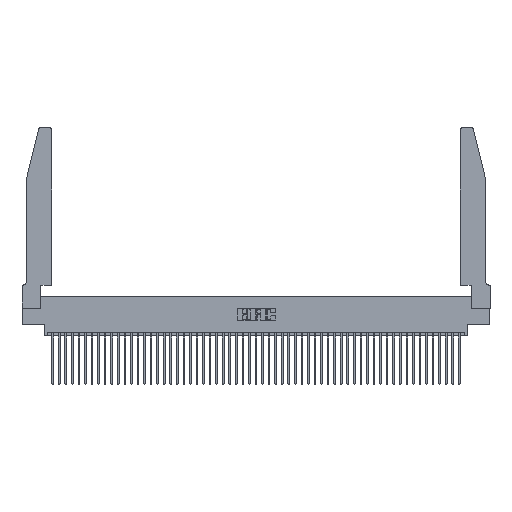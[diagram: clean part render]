
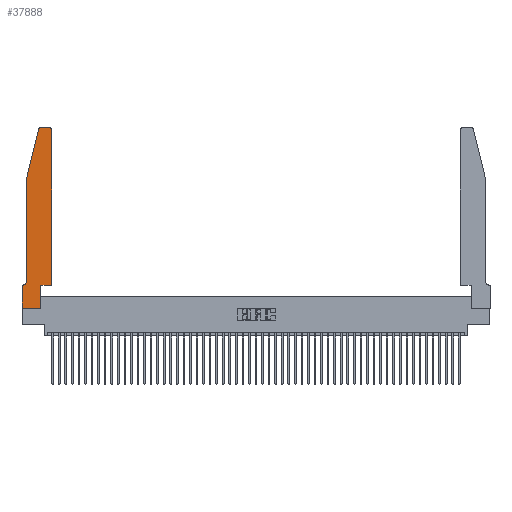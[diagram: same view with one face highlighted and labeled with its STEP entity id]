
A CAD part, top view. The second image highlights one B-rep face of the part: STEP entity #37888.
In plain terms, the highlighted planar face has unit normal (0, 0, 1).
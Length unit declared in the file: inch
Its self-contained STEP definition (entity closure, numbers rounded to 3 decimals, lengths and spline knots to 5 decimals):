
#162 = CARTESIAN_POINT ( 'NONE',  ( 0., 0.35, 0.37 ) ) ;
#283 = VERTEX_POINT ( 'NONE', #8552 ) ;
#716 = VECTOR ( 'NONE', #48132, 39.37008 ) ;
#825 = CARTESIAN_POINT ( 'NONE',  ( 0.25487, 2.72718, 0.37 ) ) ;
#1293 = DIRECTION ( 'NONE',  ( 0., -1., 0. ) ) ;
#2922 = VECTOR ( 'NONE', #34797, 39.37008 ) ;
#3136 = EDGE_CURVE ( 'NONE', #283, #15761, #44044, .T. ) ;
#3512 = VERTEX_POINT ( 'NONE', #41169 ) ;
#4586 = CARTESIAN_POINT ( 'NONE',  ( 0.4505, 0.35, 0.37 ) ) ;
#4816 = AXIS2_PLACEMENT_3D ( 'NONE', #5595, #33410, #9637 ) ;
#4942 = ORIENTED_EDGE ( 'NONE', *, *, #33580, .T. ) ;
#4998 = EDGE_LOOP ( 'NONE', ( #26605, #4942, #18418, #17762, #19872, #23298, #47018, #38836, #42365, #28641, #6036, #6969 ) ) ;
#5595 = CARTESIAN_POINT ( 'NONE',  ( 0.4205, 2.72, 0.37 ) ) ;
#5691 = EDGE_CURVE ( 'NONE', #38241, #20779, #33320, .T. ) ;
#6036 = ORIENTED_EDGE ( 'NONE', *, *, #36474, .T. ) ;
#6043 = DIRECTION ( 'NONE',  ( 1., 0., 0. ) ) ;
#6724 = EDGE_CURVE ( 'NONE', #15507, #38241, #8358, .T. ) ;
#6803 = CARTESIAN_POINT ( 'NONE',  ( 0.0755, 2., 0.37 ) ) ;
#6969 = ORIENTED_EDGE ( 'NONE', *, *, #6724, .T. ) ;
#8358 = CIRCLE ( 'NONE', #4816, 0.03 ) ;
#8552 = CARTESIAN_POINT ( 'NONE',  ( 0.0055, 0.35, 0.37 ) ) ;
#9637 = DIRECTION ( 'NONE',  ( 1., 0., 0. ) ) ;
#11343 = DIRECTION ( 'NONE',  ( 0., 0., 1. ) ) ;
#11778 = AXIS2_PLACEMENT_3D ( 'NONE', #40588, #16856, #44580 ) ;
#12446 = VECTOR ( 'NONE', #27207, 39.37008 ) ;
#14537 = VERTEX_POINT ( 'NONE', #825 ) ;
#14762 = CARTESIAN_POINT ( 'NONE',  ( 0.2865, 0., 0.37 ) ) ;
#15507 = VERTEX_POINT ( 'NONE', #30816 ) ;
#15639 = VECTOR ( 'NONE', #36257, 39.37008 ) ;
#15725 = AXIS2_PLACEMENT_3D ( 'NONE', #19153, #46863, #23155 ) ;
#15761 = VERTEX_POINT ( 'NONE', #162 ) ;
#16856 = DIRECTION ( 'NONE',  ( 0., 0., 1. ) ) ;
#17279 = CARTESIAN_POINT ( 'NONE',  ( 0.0755, 2., 0.37 ) ) ;
#17762 = ORIENTED_EDGE ( 'NONE', *, *, #49974, .T. ) ;
#17944 = LINE ( 'NONE', #29884, #28531 ) ;
#18418 = ORIENTED_EDGE ( 'NONE', *, *, #46883, .T. ) ;
#19153 = CARTESIAN_POINT ( 'NONE',  ( 0.0055, 0.42, 0.37 ) ) ;
#19299 = VERTEX_POINT ( 'NONE', #21477 ) ;
#19872 = ORIENTED_EDGE ( 'NONE', *, *, #39367, .T. ) ;
#20323 = LINE ( 'NONE', #31313, #29661 ) ;
#20645 = FACE_OUTER_BOUND ( 'NONE', #4998, .T. ) ;
#20779 = VERTEX_POINT ( 'NONE', #38703 ) ;
#21477 = CARTESIAN_POINT ( 'NONE',  ( 0.0755, 2., 0.37 ) ) ;
#22105 = EDGE_CURVE ( 'NONE', #25375, #26283, #17944, .T. ) ;
#23155 = DIRECTION ( 'NONE',  ( -1., 0., 0. ) ) ;
#23298 = ORIENTED_EDGE ( 'NONE', *, *, #3136, .T. ) ;
#23300 = DIRECTION ( 'NONE',  ( 0., -1., 0. ) ) ;
#25375 = VERTEX_POINT ( 'NONE', #35453 ) ;
#25860 = VERTEX_POINT ( 'NONE', #14762 ) ;
#26176 = LINE ( 'NONE', #47961, #15639 ) ;
#26283 = VERTEX_POINT ( 'NONE', #49134 ) ;
#26605 = ORIENTED_EDGE ( 'NONE', *, *, #5691, .T. ) ;
#27036 = VECTOR ( 'NONE', #1293, 39.37008 ) ;
#27207 = DIRECTION ( 'NONE',  ( -1., 0., 0. ) ) ;
#27300 = DIRECTION ( 'NONE',  ( -1., 0., 0. ) ) ;
#28531 = VECTOR ( 'NONE', #6043, 39.37008 ) ;
#28641 = ORIENTED_EDGE ( 'NONE', *, *, #22105, .T. ) ;
#29661 = VECTOR ( 'NONE', #23300, 39.37008 ) ;
#29884 = CARTESIAN_POINT ( 'NONE',  ( 0.4505, 0.35, 0.37 ) ) ;
#30406 = CARTESIAN_POINT ( 'NONE',  ( 0., 0., 0.37 ) ) ;
#30816 = CARTESIAN_POINT ( 'NONE',  ( 0.4505, 2.72, 0.37 ) ) ;
#31076 = CIRCLE ( 'NONE', #35219, 0.03 ) ;
#31313 = CARTESIAN_POINT ( 'NONE',  ( 0., 0., 0.37 ) ) ;
#32307 = EDGE_CURVE ( 'NONE', #25860, #25375, #26176, .T. ) ;
#32635 = VECTOR ( 'NONE', #34393, 39.37008 ) ;
#33320 = LINE ( 'NONE', #50922, #42599 ) ;
#33410 = DIRECTION ( 'NONE',  ( 0., 0., 1. ) ) ;
#33475 = LINE ( 'NONE', #6803, #2922 ) ;
#33580 = EDGE_CURVE ( 'NONE', #20779, #14537, #31076, .T. ) ;
#34393 = DIRECTION ( 'NONE',  ( 1., 0., 0. ) ) ;
#34797 = DIRECTION ( 'NONE',  ( -0.239, -0.971, 0. ) ) ;
#35069 = CARTESIAN_POINT ( 'NONE',  ( 0.284, 2.72, 0.37 ) ) ;
#35219 = AXIS2_PLACEMENT_3D ( 'NONE', #35069, #11343, #39059 ) ;
#35453 = CARTESIAN_POINT ( 'NONE',  ( 0.2865, 0.35, 0.37 ) ) ;
#36257 = DIRECTION ( 'NONE',  ( 0., 1., 0. ) ) ;
#36474 = EDGE_CURVE ( 'NONE', #26283, #15507, #41870, .T. ) ;
#36648 = PLANE ( 'NONE',  #11778 ) ;
#37888 = ADVANCED_FACE ( 'NONE', ( #20645 ), #36648, .T. ) ;
#38095 = LINE ( 'NONE', #17279, #27036 ) ;
#38241 = VERTEX_POINT ( 'NONE', #47636 ) ;
#38703 = CARTESIAN_POINT ( 'NONE',  ( 0.284, 2.75, 0.37 ) ) ;
#38836 = ORIENTED_EDGE ( 'NONE', *, *, #48938, .T. ) ;
#39059 = DIRECTION ( 'NONE',  ( 1., 0., 0. ) ) ;
#39367 = EDGE_CURVE ( 'NONE', #43845, #283, #48710, .T. ) ;
#40588 = CARTESIAN_POINT ( 'NONE',  ( 0., 0.35, 0.37 ) ) ;
#41169 = CARTESIAN_POINT ( 'NONE',  ( 0., 0., 0.37 ) ) ;
#41270 = CARTESIAN_POINT ( 'NONE',  ( 0.0755, 0.42, 0.37 ) ) ;
#41870 = LINE ( 'NONE', #4586, #716 ) ;
#42365 = ORIENTED_EDGE ( 'NONE', *, *, #32307, .T. ) ;
#42599 = VECTOR ( 'NONE', #27300, 39.37008 ) ;
#43845 = VERTEX_POINT ( 'NONE', #41270 ) ;
#44044 = LINE ( 'NONE', #50847, #12446 ) ;
#44392 = LINE ( 'NONE', #30406, #32635 ) ;
#44580 = DIRECTION ( 'NONE',  ( 1., 0., 0. ) ) ;
#45007 = EDGE_CURVE ( 'NONE', #15761, #3512, #20323, .T. ) ;
#46863 = DIRECTION ( 'NONE',  ( 0., 0., -1. ) ) ;
#46883 = EDGE_CURVE ( 'NONE', #14537, #19299, #33475, .T. ) ;
#47018 = ORIENTED_EDGE ( 'NONE', *, *, #45007, .T. ) ;
#47636 = CARTESIAN_POINT ( 'NONE',  ( 0.4205, 2.75, 0.37 ) ) ;
#47961 = CARTESIAN_POINT ( 'NONE',  ( 0.2865, 0.35, 0.37 ) ) ;
#48132 = DIRECTION ( 'NONE',  ( 0., 1., 0. ) ) ;
#48710 = CIRCLE ( 'NONE', #15725, 0.07 ) ;
#48938 = EDGE_CURVE ( 'NONE', #3512, #25860, #44392, .T. ) ;
#49134 = CARTESIAN_POINT ( 'NONE',  ( 0.4505, 0.35, 0.37 ) ) ;
#49974 = EDGE_CURVE ( 'NONE', #19299, #43845, #38095, .T. ) ;
#50847 = CARTESIAN_POINT ( 'NONE',  ( 0.0755, 0.35, 0.37 ) ) ;
#50922 = CARTESIAN_POINT ( 'NONE',  ( 0.2605, 2.75, 0.37 ) ) ;
